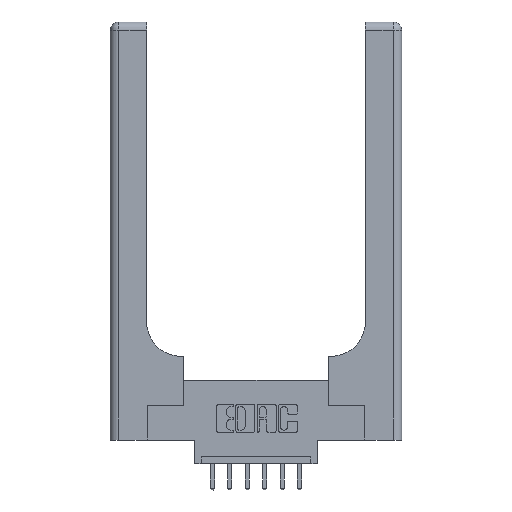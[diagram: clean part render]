
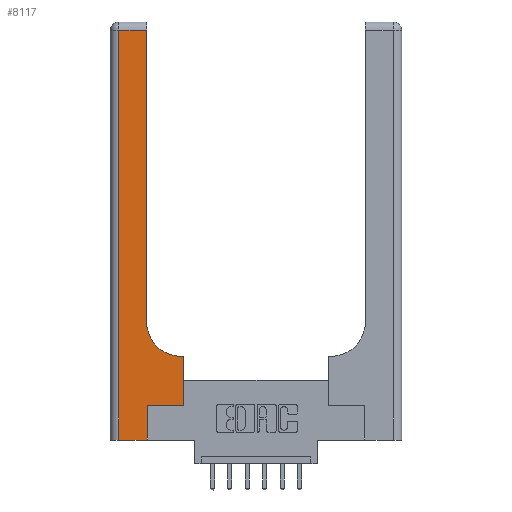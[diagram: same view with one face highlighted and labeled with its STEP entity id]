
A CAD part, top view. The second image highlights one B-rep face of the part: STEP entity #8117.
In plain terms, the highlighted planar face has unit normal (0, 0, 1).
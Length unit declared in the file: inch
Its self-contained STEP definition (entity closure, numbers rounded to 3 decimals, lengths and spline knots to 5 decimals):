
#458 = LINE ( 'NONE', #13898, #7035 ) ;
#524 = EDGE_CURVE ( 'NONE', #12842, #6003, #8872, .T. ) ;
#872 = CARTESIAN_POINT ( 'NONE',  ( 0., 2.94, 0.37 ) ) ;
#940 = CARTESIAN_POINT ( 'NONE',  ( 0.265, 0., 0.37 ) ) ;
#1205 = EDGE_CURVE ( 'NONE', #11538, #3490, #458, .T. ) ;
#1306 = EDGE_CURVE ( 'NONE', #6003, #10869, #4068, .T. ) ;
#1428 = CARTESIAN_POINT ( 'NONE',  ( 0.528, 0.6, 0.37 ) ) ;
#1832 = VERTEX_POINT ( 'NONE', #1428 ) ;
#1862 = ORIENTED_EDGE ( 'NONE', *, *, #12424, .T. ) ;
#1909 = CARTESIAN_POINT ( 'NONE',  ( 0., 0., 0.37 ) ) ;
#1910 = CARTESIAN_POINT ( 'NONE',  ( 0.51, 0.85, 0.37 ) ) ;
#2079 = CARTESIAN_POINT ( 'NONE',  ( 0.528, 0.25, 0.37 ) ) ;
#2094 = LINE ( 'NONE', #940, #10183 ) ;
#2412 = ORIENTED_EDGE ( 'NONE', *, *, #14219, .T. ) ;
#2631 = VECTOR ( 'NONE', #14293, 39.37008 ) ;
#2844 = ORIENTED_EDGE ( 'NONE', *, *, #12699, .T. ) ;
#3064 = DIRECTION ( 'NONE',  ( -1., 0., 0. ) ) ;
#3134 = ORIENTED_EDGE ( 'NONE', *, *, #524, .T. ) ;
#3301 = DIRECTION ( 'NONE',  ( -1., 0., 0. ) ) ;
#3490 = VERTEX_POINT ( 'NONE', #4219 ) ;
#3518 = CARTESIAN_POINT ( 'NONE',  ( 0.06, 2.94, 0.37 ) ) ;
#3846 = CARTESIAN_POINT ( 'NONE',  ( 0., 3., 0.37 ) ) ;
#4053 = VECTOR ( 'NONE', #5207, 39.37008 ) ;
#4068 = LINE ( 'NONE', #1909, #9398 ) ;
#4099 = DIRECTION ( 'NONE',  ( 1., 0., 0. ) ) ;
#4188 = LINE ( 'NONE', #872, #13013 ) ;
#4219 = CARTESIAN_POINT ( 'NONE',  ( 0.26, 2.94, 0.37 ) ) ;
#4678 = CARTESIAN_POINT ( 'NONE',  ( 0.26, 0.85, 0.37 ) ) ;
#5207 = DIRECTION ( 'NONE',  ( 0., -1., 0. ) ) ;
#5260 = ORIENTED_EDGE ( 'NONE', *, *, #1306, .T. ) ;
#5293 = CARTESIAN_POINT ( 'NONE',  ( 0.06, 3., 0.37 ) ) ;
#5361 = CARTESIAN_POINT ( 'NONE',  ( 0.265, 0.25, 0.37 ) ) ;
#5378 = DIRECTION ( 'NONE',  ( 0., 1., 0. ) ) ;
#5568 = ORIENTED_EDGE ( 'NONE', *, *, #12430, .T. ) ;
#5808 = AXIS2_PLACEMENT_3D ( 'NONE', #3846, #6194, #3064 ) ;
#6003 = VERTEX_POINT ( 'NONE', #6204 ) ;
#6082 = EDGE_CURVE ( 'NONE', #7545, #11538, #11590, .T. ) ;
#6194 = DIRECTION ( 'NONE',  ( 0., 0., -1. ) ) ;
#6204 = CARTESIAN_POINT ( 'NONE',  ( 0.06, 0., 0.37 ) ) ;
#7035 = VECTOR ( 'NONE', #10666, 39.37008 ) ;
#7354 = VECTOR ( 'NONE', #3301, 39.37008 ) ;
#7445 = FACE_OUTER_BOUND ( 'NONE', #11437, .T. ) ;
#7545 = VERTEX_POINT ( 'NONE', #10521 ) ;
#7740 = CARTESIAN_POINT ( 'NONE',  ( 0.265, 0.25, 0.37 ) ) ;
#7814 = LINE ( 'NONE', #13333, #7354 ) ;
#8117 = ADVANCED_FACE ( 'NONE', ( #7445 ), #9483, .F. ) ;
#8149 = CARTESIAN_POINT ( 'NONE',  ( 0.265, 0., 0.37 ) ) ;
#8668 = DIRECTION ( 'NONE',  ( -1., 0., 0. ) ) ;
#8872 = LINE ( 'NONE', #5293, #4053 ) ;
#9054 = ORIENTED_EDGE ( 'NONE', *, *, #6082, .T. ) ;
#9104 = VERTEX_POINT ( 'NONE', #7740 ) ;
#9398 = VECTOR ( 'NONE', #13245, 39.37008 ) ;
#9483 = PLANE ( 'NONE',  #5808 ) ;
#10183 = VECTOR ( 'NONE', #5378, 39.37008 ) ;
#10249 = EDGE_CURVE ( 'NONE', #9104, #12064, #10834, .T. ) ;
#10442 = DIRECTION ( 'NONE',  ( 0., 0., -1. ) ) ;
#10521 = CARTESIAN_POINT ( 'NONE',  ( 0.51, 0.6, 0.37 ) ) ;
#10666 = DIRECTION ( 'NONE',  ( 0., 1., 0. ) ) ;
#10834 = LINE ( 'NONE', #5361, #10952 ) ;
#10835 = LINE ( 'NONE', #2079, #2631 ) ;
#10869 = VERTEX_POINT ( 'NONE', #8149 ) ;
#10952 = VECTOR ( 'NONE', #4099, 39.37008 ) ;
#11437 = EDGE_LOOP ( 'NONE', ( #12604, #1862, #3134, #5260, #5568, #13402, #2844, #2412, #9054 ) ) ;
#11538 = VERTEX_POINT ( 'NONE', #4678 ) ;
#11590 = CIRCLE ( 'NONE', #13490, 0.25 ) ;
#12064 = VERTEX_POINT ( 'NONE', #13094 ) ;
#12424 = EDGE_CURVE ( 'NONE', #3490, #12842, #4188, .T. ) ;
#12430 = EDGE_CURVE ( 'NONE', #10869, #9104, #2094, .T. ) ;
#12604 = ORIENTED_EDGE ( 'NONE', *, *, #1205, .T. ) ;
#12699 = EDGE_CURVE ( 'NONE', #12064, #1832, #10835, .T. ) ;
#12820 = DIRECTION ( 'NONE',  ( 1., 0., 0. ) ) ;
#12842 = VERTEX_POINT ( 'NONE', #3518 ) ;
#13013 = VECTOR ( 'NONE', #8668, 39.37008 ) ;
#13094 = CARTESIAN_POINT ( 'NONE',  ( 0.528, 0.25, 0.37 ) ) ;
#13245 = DIRECTION ( 'NONE',  ( 1., 0., 0. ) ) ;
#13333 = CARTESIAN_POINT ( 'NONE',  ( 0.26, 0.6, 0.37 ) ) ;
#13402 = ORIENTED_EDGE ( 'NONE', *, *, #10249, .T. ) ;
#13490 = AXIS2_PLACEMENT_3D ( 'NONE', #1910, #10442, #12820 ) ;
#13898 = CARTESIAN_POINT ( 'NONE',  ( 0.26, 3., 0.37 ) ) ;
#14219 = EDGE_CURVE ( 'NONE', #1832, #7545, #7814, .T. ) ;
#14293 = DIRECTION ( 'NONE',  ( 0., 1., 0. ) ) ;
